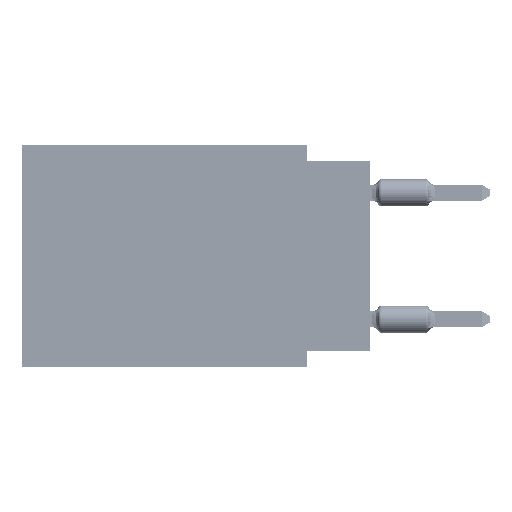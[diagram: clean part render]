
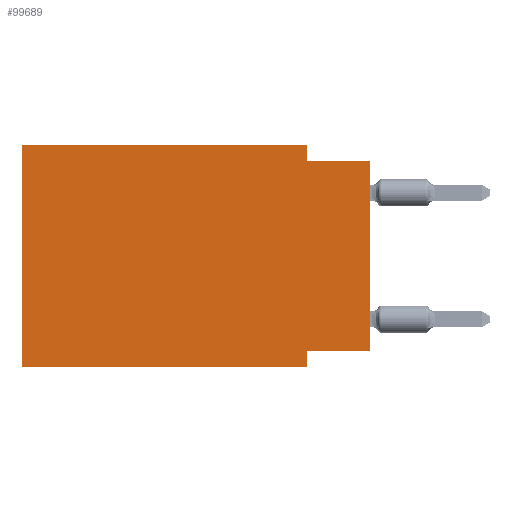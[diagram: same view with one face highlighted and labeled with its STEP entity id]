
A CAD part, left-side view. The second image highlights one B-rep face of the part: STEP entity #99689.
In plain terms, the highlighted planar face has unit normal (-1, 0, 0).
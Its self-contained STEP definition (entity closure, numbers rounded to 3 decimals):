
#1026 = VECTOR ( 'NONE', #5903, 1000. ) ;
#2477 = VECTOR ( 'NONE', #46757, 1000. ) ;
#3190 = CARTESIAN_POINT ( 'NONE',  ( 0., 13.97, 0. ) ) ;
#3766 = VERTEX_POINT ( 'NONE', #49608 ) ;
#5903 = DIRECTION ( 'NONE',  ( 0., -1., 0. ) ) ;
#8551 = VECTOR ( 'NONE', #26576, 1000. ) ;
#9181 = AXIS2_PLACEMENT_3D ( 'NONE', #98230, #10899, #50426 ) ;
#9270 = CARTESIAN_POINT ( 'NONE',  ( 0., 2.54, -8.255 ) ) ;
#9383 = VECTOR ( 'NONE', #90148, 1000. ) ;
#9643 = LINE ( 'NONE', #40454, #8551 ) ;
#10899 = DIRECTION ( 'NONE',  ( 1., 0., 0. ) ) ;
#14906 = VERTEX_POINT ( 'NONE', #35942 ) ;
#15369 = VECTOR ( 'NONE', #101050, 1000. ) ;
#15998 = VERTEX_POINT ( 'NONE', #59845 ) ;
#17612 = VERTEX_POINT ( 'NONE', #9270 ) ;
#19089 = PLANE ( 'NONE',  #9181 ) ;
#22100 = DIRECTION ( 'NONE',  ( 0., -1., 0. ) ) ;
#26084 = EDGE_CURVE ( 'NONE', #14906, #3766, #57650, .T. ) ;
#26128 = EDGE_CURVE ( 'NONE', #96042, #81913, #93545, .T. ) ;
#26576 = DIRECTION ( 'NONE',  ( 0., 0., 1. ) ) ;
#26924 = EDGE_CURVE ( 'NONE', #17612, #33491, #89647, .T. ) ;
#28115 = ORIENTED_EDGE ( 'NONE', *, *, #26084, .F. ) ;
#30056 = LINE ( 'NONE', #69620, #1026 ) ;
#30285 = LINE ( 'NONE', #37475, #78538 ) ;
#30633 = ORIENTED_EDGE ( 'NONE', *, *, #26128, .F. ) ;
#33491 = VERTEX_POINT ( 'NONE', #38346 ) ;
#35942 = CARTESIAN_POINT ( 'NONE',  ( 0., 13.97, -8.89 ) ) ;
#37475 = CARTESIAN_POINT ( 'NONE',  ( 0., 2.54, 0. ) ) ;
#37708 = EDGE_CURVE ( 'NONE', #15998, #17612, #55781, .T. ) ;
#37963 = ORIENTED_EDGE ( 'NONE', *, *, #26924, .F. ) ;
#38346 = CARTESIAN_POINT ( 'NONE',  ( 0., 2.54, -8.89 ) ) ;
#38821 = CARTESIAN_POINT ( 'NONE',  ( 0., 0., -8.255 ) ) ;
#40293 = VECTOR ( 'NONE', #22100, 1000. ) ;
#40454 = CARTESIAN_POINT ( 'NONE',  ( 0., 0., 0. ) ) ;
#44170 = EDGE_CURVE ( 'NONE', #3766, #98336, #69393, .T. ) ;
#46757 = DIRECTION ( 'NONE',  ( 0., -1., 0. ) ) ;
#49608 = CARTESIAN_POINT ( 'NONE',  ( 0., 13.97, 0. ) ) ;
#50035 = ORIENTED_EDGE ( 'NONE', *, *, #37708, .F. ) ;
#50426 = DIRECTION ( 'NONE',  ( 0., 0., -1. ) ) ;
#51569 = ORIENTED_EDGE ( 'NONE', *, *, #54135, .T. ) ;
#54135 = EDGE_CURVE ( 'NONE', #14906, #33491, #30056, .T. ) ;
#55781 = LINE ( 'NONE', #38821, #15369 ) ;
#55885 = ORIENTED_EDGE ( 'NONE', *, *, #58689, .F. ) ;
#57650 = LINE ( 'NONE', #3190, #76300 ) ;
#58689 = EDGE_CURVE ( 'NONE', #98336, #96042, #30285, .T. ) ;
#58792 = CARTESIAN_POINT ( 'NONE',  ( 0., 2.54, -8.89 ) ) ;
#59845 = CARTESIAN_POINT ( 'NONE',  ( 0., 0., -8.255 ) ) ;
#60653 = CARTESIAN_POINT ( 'NONE',  ( 0., 0., -0.635 ) ) ;
#64098 = EDGE_CURVE ( 'NONE', #15998, #81913, #9643, .T. ) ;
#64340 = CARTESIAN_POINT ( 'NONE',  ( 0., 2.54, 0. ) ) ;
#64851 = CARTESIAN_POINT ( 'NONE',  ( 0., 0., -0.635 ) ) ;
#66862 = DIRECTION ( 'NONE',  ( 0., 0., 1. ) ) ;
#68614 = ORIENTED_EDGE ( 'NONE', *, *, #44170, .F. ) ;
#69393 = LINE ( 'NONE', #99741, #40293 ) ;
#69620 = CARTESIAN_POINT ( 'NONE',  ( 0., 13.97, -8.89 ) ) ;
#69791 = ORIENTED_EDGE ( 'NONE', *, *, #64098, .T. ) ;
#76300 = VECTOR ( 'NONE', #66862, 1000. ) ;
#78538 = VECTOR ( 'NONE', #98691, 1000. ) ;
#79205 = EDGE_LOOP ( 'NONE', ( #69791, #30633, #55885, #68614, #28115, #51569, #37963, #50035 ) ) ;
#81297 = FACE_OUTER_BOUND ( 'NONE', #79205, .T. ) ;
#81913 = VERTEX_POINT ( 'NONE', #64851 ) ;
#89647 = LINE ( 'NONE', #58792, #9383 ) ;
#90148 = DIRECTION ( 'NONE',  ( 0., 0., -1. ) ) ;
#93545 = LINE ( 'NONE', #60653, #2477 ) ;
#96042 = VERTEX_POINT ( 'NONE', #97122 ) ;
#97122 = CARTESIAN_POINT ( 'NONE',  ( 0., 2.54, -0.635 ) ) ;
#98230 = CARTESIAN_POINT ( 'NONE',  ( 0., 13.97, 0. ) ) ;
#98336 = VERTEX_POINT ( 'NONE', #64340 ) ;
#98691 = DIRECTION ( 'NONE',  ( 0., 0., -1. ) ) ;
#99689 = ADVANCED_FACE ( 'NONE', ( #81297 ), #19089, .F. ) ;
#99741 = CARTESIAN_POINT ( 'NONE',  ( 0., 13.97, 0. ) ) ;
#101050 = DIRECTION ( 'NONE',  ( 0., 1., 0. ) ) ;
